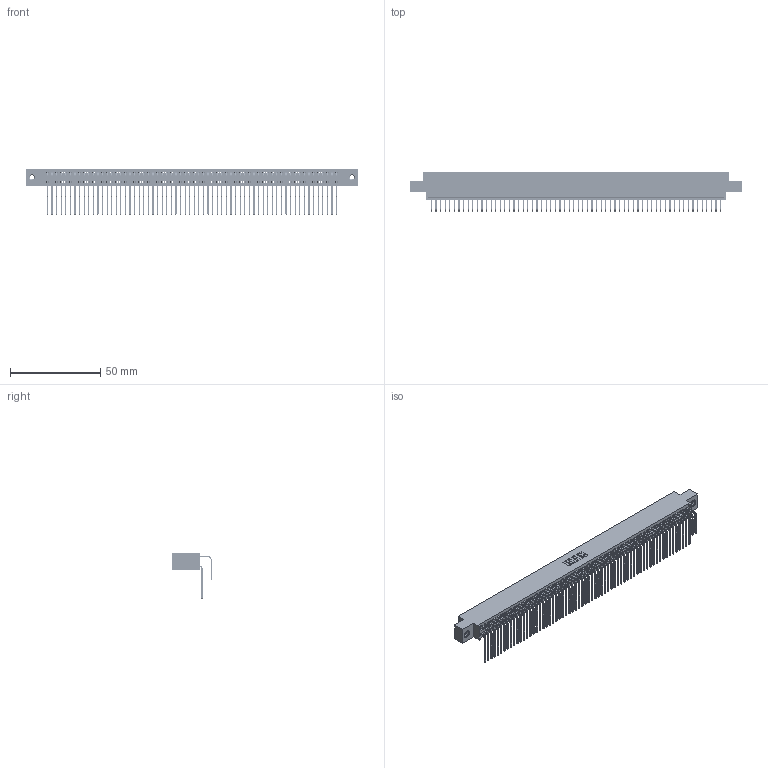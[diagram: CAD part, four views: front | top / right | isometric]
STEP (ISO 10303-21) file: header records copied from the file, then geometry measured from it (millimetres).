
FILE_DESCRIPTION (( 'STEP AP203' ), '1' );
FILE_NAME ('395-128-558-808.STEP', '2018-12-04T13:48:23', ( '' ), ( '' ), 'SwSTEP 2.0', 'SolidWorks 2016', '' );
FILE_SCHEMA (( 'CONFIG_CONTROL_DESIGN' ));
Length unit declared in the file: inch
Products named in the file (5): 395-128-558-808; 345 Part_0.170 Offset - 0.156 Dia-TI; 345-250-001_345-250-003-102; 345-292-001_558 559 Tail - 1; 345-292-001_558 Tail - 2
Assembly tree (131 placements, depth 2):
  395-128-558-808
    345 Part_0.170 Offset - 0.156 Dia-TI
    345-292-001_558 559 Tail - 1  x64
    345-292-001_558 Tail - 2  x64
    345-250-001_345-250-003-102  x2
Bounding box: 183.77 x 21.83 x 25.53 mm (x, y, z)
Volume: 18674.2 mm3; surface area: 31658.8 mm2
Topology: 131 solids, 131 shells, 6846 faces, 20329 edges, 13374 vertices
Faces by surface type: plane 4596, cylinder 2234, cone 12, torus 4
Entity records: 50224 total; most frequent: CARTESIAN_POINT 8426, ORIENTED_EDGE 8302, DIRECTION 7401, EDGE_CURVE 4151, LINE 3703, VECTOR 3703, VERTEX_POINT 2760, AXIS2_PLACEMENT_3D 1849
